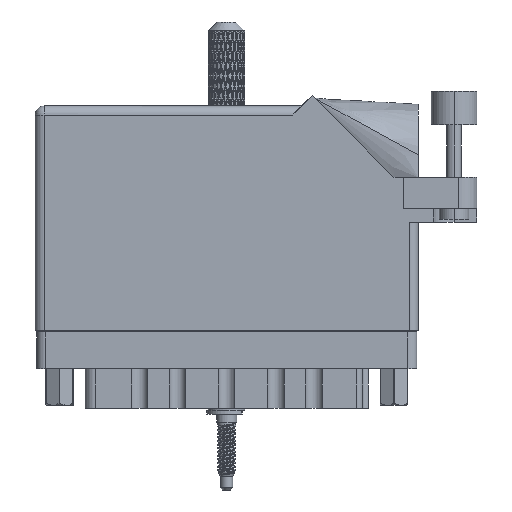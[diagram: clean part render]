
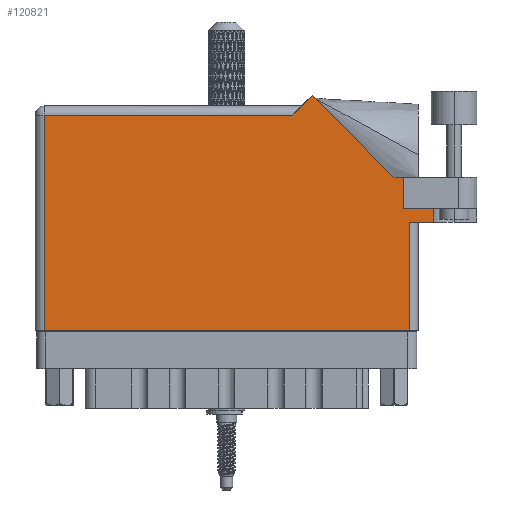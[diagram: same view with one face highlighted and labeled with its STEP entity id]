
A CAD part, front view. The second image highlights one B-rep face of the part: STEP entity #120821.
In plain terms, the highlighted face is planar.
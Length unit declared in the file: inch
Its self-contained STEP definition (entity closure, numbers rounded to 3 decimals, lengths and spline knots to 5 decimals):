
#1317 = CARTESIAN_POINT ( 'NONE',  ( 3.012, 1.044, 0. ) ) ;
#3094 = VERTEX_POINT ( 'NONE', #82496 ) ;
#5640 = ORIENTED_EDGE ( 'NONE', *, *, #40047, .T. ) ;
#6133 = VERTEX_POINT ( 'NONE', #51954 ) ;
#7434 = VECTOR ( 'NONE', #56241, 39.37008 ) ;
#8444 = VERTEX_POINT ( 'NONE', #114877 ) ;
#8625 = CARTESIAN_POINT ( 'NONE',  ( 0., 1.468, 0. ) ) ;
#8789 = ORIENTED_EDGE ( 'NONE', *, *, #106958, .T. ) ;
#9231 = LINE ( 'NONE', #104637, #112373 ) ;
#10213 = VERTEX_POINT ( 'NONE', #48083 ) ;
#10840 = DIRECTION ( 'NONE',  ( 1., 0., 0. ) ) ;
#14151 = LINE ( 'NONE', #117911, #72465 ) ;
#16869 = VERTEX_POINT ( 'NONE', #26471 ) ;
#19128 = VECTOR ( 'NONE', #76817, 39.37008 ) ;
#20313 = CARTESIAN_POINT ( 'NONE',  ( 2.512, 0.831, 0. ) ) ;
#20609 = VECTOR ( 'NONE', #10840, 39.37008 ) ;
#21285 = EDGE_CURVE ( 'NONE', #3094, #98092, #53646, .T. ) ;
#21636 = EDGE_CURVE ( 'NONE', #8444, #3094, #62578, .T. ) ;
#22584 = EDGE_CURVE ( 'NONE', #98092, #6133, #117796, .T. ) ;
#23995 = LINE ( 'NONE', #20313, #7434 ) ;
#25816 = AXIS2_PLACEMENT_3D ( 'NONE', #96681, #86271, #77896 ) ;
#26381 = DIRECTION ( 'NONE',  ( -0.707, 0.707, 0. ) ) ;
#26471 = CARTESIAN_POINT ( 'NONE',  ( 2.7135, 0.831, 0. ) ) ;
#27093 = DIRECTION ( 'NONE',  ( 1., 0., 0. ) ) ;
#28700 = VECTOR ( 'NONE', #108926, 39.37008 ) ;
#29719 = VERTEX_POINT ( 'NONE', #73018 ) ;
#30097 = CARTESIAN_POINT ( 'NONE',  ( 2.612, 0.737, 0. ) ) ;
#30257 = FACE_OUTER_BOUND ( 'NONE', #104577, .T. ) ;
#32570 = VERTEX_POINT ( 'NONE', #78023 ) ;
#34273 = LINE ( 'NONE', #55993, #116457 ) ;
#34837 = EDGE_CURVE ( 'NONE', #16869, #29719, #9231, .T. ) ;
#35686 = VECTOR ( 'NONE', #108439, 39.37008 ) ;
#36756 = ORIENTED_EDGE ( 'NONE', *, *, #102334, .T. ) ;
#37343 = EDGE_CURVE ( 'NONE', #91510, #104728, #34273, .T. ) ;
#40047 = EDGE_CURVE ( 'NONE', #78312, #91510, #54826, .T. ) ;
#46798 = CARTESIAN_POINT ( 'NONE',  ( 0.062, 0., 0. ) ) ;
#48083 = CARTESIAN_POINT ( 'NONE',  ( 2.55, 0.737, 0. ) ) ;
#49990 = ORIENTED_EDGE ( 'NONE', *, *, #21285, .T. ) ;
#50860 = CARTESIAN_POINT ( 'NONE',  ( 2.512, 0.831, 0. ) ) ;
#51954 = CARTESIAN_POINT ( 'NONE',  ( 2.55, 0., 0. ) ) ;
#53646 = LINE ( 'NONE', #106302, #35686 ) ;
#54826 = LINE ( 'NONE', #1317, #59219 ) ;
#55993 = CARTESIAN_POINT ( 'NONE',  ( 2.44642, 1.044, 0. ) ) ;
#56213 = ORIENTED_EDGE ( 'NONE', *, *, #21636, .T. ) ;
#56241 = DIRECTION ( 'NONE',  ( 0., 1., 0. ) ) ;
#59219 = VECTOR ( 'NONE', #77083, 39.37008 ) ;
#62578 = LINE ( 'NONE', #8625, #19128 ) ;
#64199 = EDGE_CURVE ( 'NONE', #32570, #16869, #122035, .T. ) ;
#67433 = CARTESIAN_POINT ( 'NONE',  ( 1.88971, 1.60071, 0. ) ) ;
#68318 = VECTOR ( 'NONE', #27093, 39.37008 ) ;
#72465 = VECTOR ( 'NONE', #98739, 39.37008 ) ;
#73018 = CARTESIAN_POINT ( 'NONE',  ( 2.7135, 0.737, 0. ) ) ;
#73438 = ORIENTED_EDGE ( 'NONE', *, *, #34837, .F. ) ;
#73629 = EDGE_CURVE ( 'NONE', #104728, #8444, #14151, .T. ) ;
#76817 = DIRECTION ( 'NONE',  ( -1., 0., 0. ) ) ;
#77083 = DIRECTION ( 'NONE',  ( -1., 0., 0. ) ) ;
#77158 = DIRECTION ( 'NONE',  ( 0., -1., 0. ) ) ;
#77896 = DIRECTION ( 'NONE',  ( -1., 0., 0. ) ) ;
#78023 = CARTESIAN_POINT ( 'NONE',  ( 2.512, 0.831, 0. ) ) ;
#78312 = VERTEX_POINT ( 'NONE', #91851 ) ;
#81732 = ORIENTED_EDGE ( 'NONE', *, *, #22584, .T. ) ;
#82496 = CARTESIAN_POINT ( 'NONE',  ( 0.062, 1.468, 0. ) ) ;
#85571 = CARTESIAN_POINT ( 'NONE',  ( 0., 0., 0. ) ) ;
#86271 = DIRECTION ( 'NONE',  ( 0., 0., -1. ) ) ;
#87079 = PLANE ( 'NONE',  #25816 ) ;
#87515 = EDGE_CURVE ( 'NONE', #32570, #78312, #23995, .T. ) ;
#88517 = DIRECTION ( 'NONE',  ( 1., 0., 0. ) ) ;
#91510 = VERTEX_POINT ( 'NONE', #108500 ) ;
#91851 = CARTESIAN_POINT ( 'NONE',  ( 2.512, 1.044, 0. ) ) ;
#95452 = ORIENTED_EDGE ( 'NONE', *, *, #64199, .F. ) ;
#96681 = CARTESIAN_POINT ( 'NONE',  ( 0., 1.53, 0. ) ) ;
#98092 = VERTEX_POINT ( 'NONE', #46798 ) ;
#98739 = DIRECTION ( 'NONE',  ( -0.707, -0.707, 0. ) ) ;
#102334 = EDGE_CURVE ( 'NONE', #6133, #10213, #115322, .T. ) ;
#104577 = EDGE_LOOP ( 'NONE', ( #81732, #36756, #8789, #73438, #95452, #106113, #5640, #123799, #107237, #56213, #49990 ) ) ;
#104637 = CARTESIAN_POINT ( 'NONE',  ( 2.7135, 1.16177, 0. ) ) ;
#104728 = VERTEX_POINT ( 'NONE', #67433 ) ;
#106113 = ORIENTED_EDGE ( 'NONE', *, *, #87515, .T. ) ;
#106302 = CARTESIAN_POINT ( 'NONE',  ( 0.062, 0., 0. ) ) ;
#106958 = EDGE_CURVE ( 'NONE', #10213, #29719, #122259, .T. ) ;
#107087 = VECTOR ( 'NONE', #88517, 39.37008 ) ;
#107216 = CARTESIAN_POINT ( 'NONE',  ( 2.55, 0.737, 0. ) ) ;
#107237 = ORIENTED_EDGE ( 'NONE', *, *, #73629, .T. ) ;
#108439 = DIRECTION ( 'NONE',  ( 0., -1., 0. ) ) ;
#108500 = CARTESIAN_POINT ( 'NONE',  ( 2.44642, 1.044, 0. ) ) ;
#108926 = DIRECTION ( 'NONE',  ( 0., 1., 0. ) ) ;
#112373 = VECTOR ( 'NONE', #77158, 39.37008 ) ;
#114877 = CARTESIAN_POINT ( 'NONE',  ( 1.757, 1.468, 0. ) ) ;
#115322 = LINE ( 'NONE', #107216, #28700 ) ;
#116457 = VECTOR ( 'NONE', #26381, 39.37008 ) ;
#117796 = LINE ( 'NONE', #85571, #68318 ) ;
#117911 = CARTESIAN_POINT ( 'NONE',  ( 1.819, 1.53, 0. ) ) ;
#120821 = ADVANCED_FACE ( 'NONE', ( #30257 ), #87079, .F. ) ;
#122035 = LINE ( 'NONE', #50860, #107087 ) ;
#122259 = LINE ( 'NONE', #30097, #20609 ) ;
#123799 = ORIENTED_EDGE ( 'NONE', *, *, #37343, .T. ) ;
